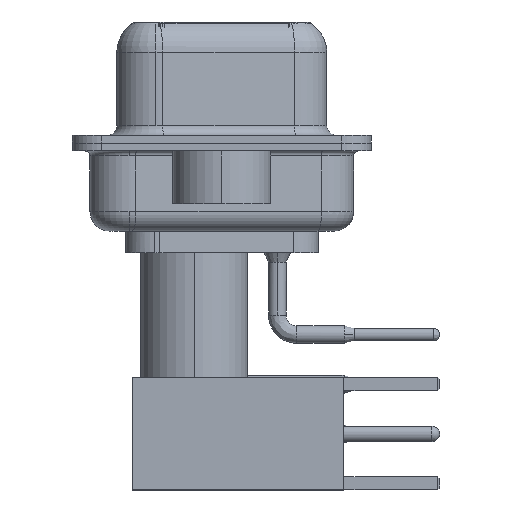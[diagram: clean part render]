
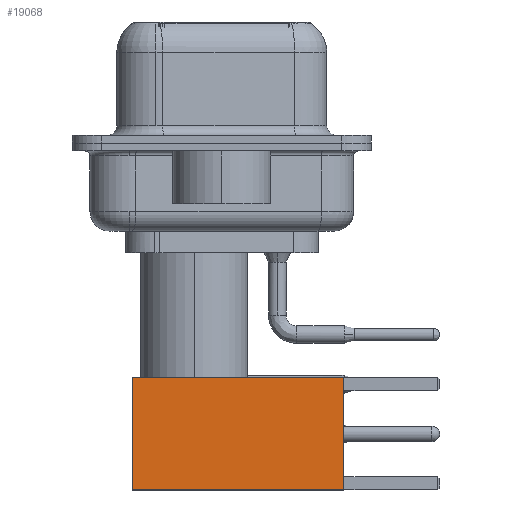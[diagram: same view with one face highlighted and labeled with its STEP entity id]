
A CAD part, left-side view. The second image highlights one B-rep face of the part: STEP entity #19068.
In plain terms, the highlighted face is planar.
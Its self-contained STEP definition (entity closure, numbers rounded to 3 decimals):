
#1292 = LINE ( 'NONE', #34917, #6061 ) ;
#2854 = ORIENTED_EDGE ( 'NONE', *, *, #31094, .F. ) ;
#6061 = VECTOR ( 'NONE', #9820, 1000. ) ;
#6167 = DIRECTION ( 'NONE',  ( 0., 0., 1. ) ) ;
#6874 = VECTOR ( 'NONE', #32477, 1000. ) ;
#7358 = EDGE_CURVE ( 'NONE', #30936, #18702, #1292, .T. ) ;
#9611 = LINE ( 'NONE', #27088, #19969 ) ;
#9820 = DIRECTION ( 'NONE',  ( 0., 0., -1. ) ) ;
#12867 = CARTESIAN_POINT ( 'NONE',  ( 2.875, 2.875, 0. ) ) ;
#15942 = CARTESIAN_POINT ( 'NONE',  ( -2.875, 2.875, 10.82 ) ) ;
#16096 = LINE ( 'NONE', #27202, #28289 ) ;
#17078 = VERTEX_POINT ( 'NONE', #15942 ) ;
#17290 = FACE_OUTER_BOUND ( 'NONE', #20464, .T. ) ;
#18702 = VERTEX_POINT ( 'NONE', #34398 ) ;
#19068 = ADVANCED_FACE ( 'NONE', ( #17290 ), #31088, .T. ) ;
#19475 = ORIENTED_EDGE ( 'NONE', *, *, #26009, .T. ) ;
#19969 = VECTOR ( 'NONE', #32525, 1000. ) ;
#20011 = DIRECTION ( 'NONE',  ( 0., 1., 0. ) ) ;
#20464 = EDGE_LOOP ( 'NONE', ( #26848, #19475, #21839, #2854 ) ) ;
#21839 = ORIENTED_EDGE ( 'NONE', *, *, #27309, .F. ) ;
#23947 = LINE ( 'NONE', #35016, #6874 ) ;
#26009 = EDGE_CURVE ( 'NONE', #18702, #35583, #16096, .T. ) ;
#26848 = ORIENTED_EDGE ( 'NONE', *, *, #7358, .T. ) ;
#27088 = CARTESIAN_POINT ( 'NONE',  ( 0., 2.875, 10.82 ) ) ;
#27202 = CARTESIAN_POINT ( 'NONE',  ( 0., 2.875, 0. ) ) ;
#27309 = EDGE_CURVE ( 'NONE', #17078, #35583, #23947, .T. ) ;
#28289 = VECTOR ( 'NONE', #35542, 1000. ) ;
#30064 = AXIS2_PLACEMENT_3D ( 'NONE', #12867, #20011, #6167 ) ;
#30936 = VERTEX_POINT ( 'NONE', #31082 ) ;
#31082 = CARTESIAN_POINT ( 'NONE',  ( 2.875, 2.875, 10.82 ) ) ;
#31088 = PLANE ( 'NONE',  #30064 ) ;
#31094 = EDGE_CURVE ( 'NONE', #30936, #17078, #9611, .T. ) ;
#32477 = DIRECTION ( 'NONE',  ( 0., 0., -1. ) ) ;
#32525 = DIRECTION ( 'NONE',  ( -1., 0., 0. ) ) ;
#34127 = CARTESIAN_POINT ( 'NONE',  ( -2.875, 2.875, 0. ) ) ;
#34398 = CARTESIAN_POINT ( 'NONE',  ( 2.875, 2.875, 0. ) ) ;
#34917 = CARTESIAN_POINT ( 'NONE',  ( 2.875, 2.875, 0. ) ) ;
#35016 = CARTESIAN_POINT ( 'NONE',  ( -2.875, 2.875, 0. ) ) ;
#35542 = DIRECTION ( 'NONE',  ( -1., 0., 0. ) ) ;
#35583 = VERTEX_POINT ( 'NONE', #34127 ) ;
